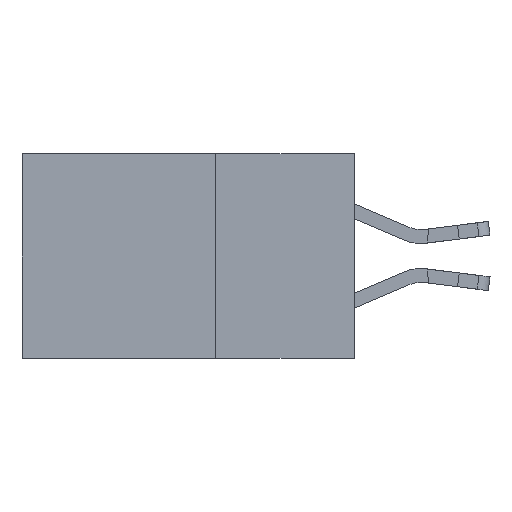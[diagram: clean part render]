
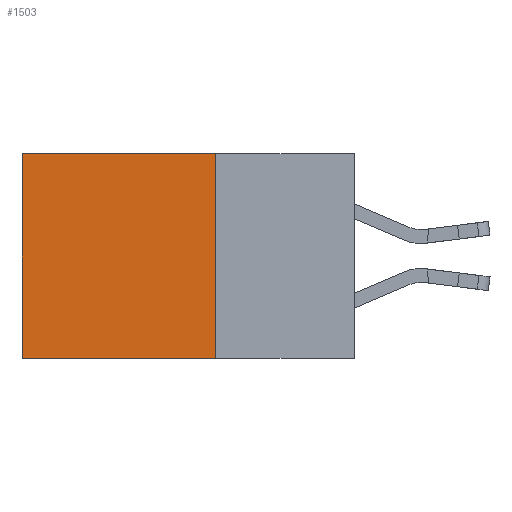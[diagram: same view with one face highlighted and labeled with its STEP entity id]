
A CAD part, left-side view. The second image highlights one B-rep face of the part: STEP entity #1503.
In plain terms, the highlighted planar face has unit normal (-1, 0, 0).
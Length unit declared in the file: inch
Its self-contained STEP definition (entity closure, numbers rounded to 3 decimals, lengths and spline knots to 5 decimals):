
#756 = EDGE_CURVE ( 'NONE', #7337, #11970, #2580, .T. ) ;
#1188 = EDGE_CURVE ( 'NONE', #11970, #6130, #3213, .T. ) ;
#1503 = ADVANCED_FACE ( 'NONE', ( #12931 ), #5206, .F. ) ;
#2008 = LINE ( 'NONE', #11139, #10242 ) ;
#2355 = VECTOR ( 'NONE', #4657, 39.37008 ) ;
#2580 = LINE ( 'NONE', #4881, #13385 ) ;
#2589 = AXIS2_PLACEMENT_3D ( 'NONE', #5811, #5129, #5148 ) ;
#3110 = ORIENTED_EDGE ( 'NONE', *, *, #1188, .F. ) ;
#3174 = CARTESIAN_POINT ( 'NONE',  ( 0.2615, 0.25, -0.37 ) ) ;
#3213 = LINE ( 'NONE', #5505, #11379 ) ;
#3439 = ORIENTED_EDGE ( 'NONE', *, *, #756, .F. ) ;
#4087 = DIRECTION ( 'NONE',  ( 0., 0., -1. ) ) ;
#4641 = CARTESIAN_POINT ( 'NONE',  ( 0.2615, 0.6, -0.37 ) ) ;
#4657 = DIRECTION ( 'NONE',  ( 0., 0., -1. ) ) ;
#4881 = CARTESIAN_POINT ( 'NONE',  ( 0.2615, 0.25, -0.37 ) ) ;
#5001 = CARTESIAN_POINT ( 'NONE',  ( 0.2615, 0.6, 0. ) ) ;
#5129 = DIRECTION ( 'NONE',  ( 1., 0., 0. ) ) ;
#5148 = DIRECTION ( 'NONE',  ( 0., 0., -1. ) ) ;
#5206 = PLANE ( 'NONE',  #2589 ) ;
#5417 = DIRECTION ( 'NONE',  ( 0., 1., 0. ) ) ;
#5505 = CARTESIAN_POINT ( 'NONE',  ( 0.2615, 0.25, -0.37 ) ) ;
#5811 = CARTESIAN_POINT ( 'NONE',  ( 0.2615, 0.25, -0.37 ) ) ;
#6130 = VERTEX_POINT ( 'NONE', #11957 ) ;
#6528 = EDGE_CURVE ( 'NONE', #8077, #6130, #8090, .T. ) ;
#6666 = ORIENTED_EDGE ( 'NONE', *, *, #7525, .T. ) ;
#7337 = VERTEX_POINT ( 'NONE', #12959 ) ;
#7525 = EDGE_CURVE ( 'NONE', #7337, #8077, #2008, .T. ) ;
#8077 = VERTEX_POINT ( 'NONE', #5001 ) ;
#8090 = LINE ( 'NONE', #4641, #2355 ) ;
#9209 = EDGE_LOOP ( 'NONE', ( #11283, #3110, #3439, #6666 ) ) ;
#10242 = VECTOR ( 'NONE', #10735, 39.37008 ) ;
#10735 = DIRECTION ( 'NONE',  ( 0., 1., 0. ) ) ;
#11139 = CARTESIAN_POINT ( 'NONE',  ( 0.2615, 0.25, 0. ) ) ;
#11283 = ORIENTED_EDGE ( 'NONE', *, *, #6528, .T. ) ;
#11379 = VECTOR ( 'NONE', #5417, 39.37008 ) ;
#11957 = CARTESIAN_POINT ( 'NONE',  ( 0.2615, 0.6, -0.37 ) ) ;
#11970 = VERTEX_POINT ( 'NONE', #3174 ) ;
#12931 = FACE_OUTER_BOUND ( 'NONE', #9209, .T. ) ;
#12959 = CARTESIAN_POINT ( 'NONE',  ( 0.2615, 0.25, 0. ) ) ;
#13385 = VECTOR ( 'NONE', #4087, 39.37008 ) ;
